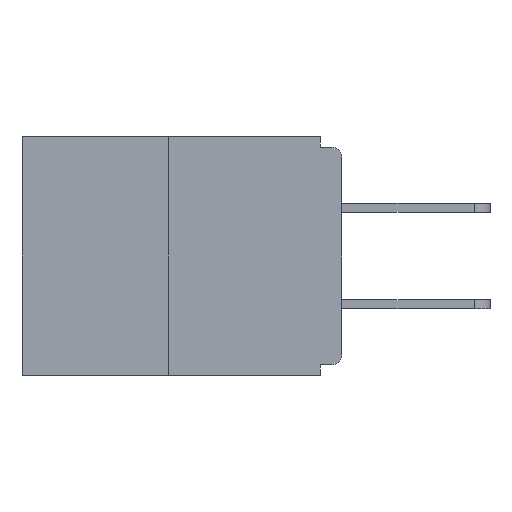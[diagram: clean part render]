
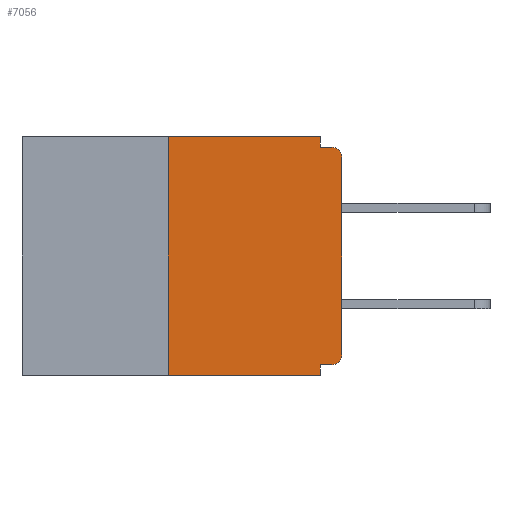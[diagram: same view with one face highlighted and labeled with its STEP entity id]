
A CAD part, left-side view. The second image highlights one B-rep face of the part: STEP entity #7056.
In plain terms, the highlighted planar face has unit normal (-1, 0, 0).
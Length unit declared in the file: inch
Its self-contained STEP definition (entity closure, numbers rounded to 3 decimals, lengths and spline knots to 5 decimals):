
#125 = VECTOR ( 'NONE', #9593, 39.37008 ) ;
#135 = CARTESIAN_POINT ( 'NONE',  ( 0., 0.25, 0. ) ) ;
#153 = ORIENTED_EDGE ( 'NONE', *, *, #1214, .F. ) ;
#228 = DIRECTION ( 'NONE',  ( 0., 0., -1. ) ) ;
#579 = VECTOR ( 'NONE', #12752, 39.37008 ) ;
#724 = VECTOR ( 'NONE', #10527, 39.37008 ) ;
#832 = VERTEX_POINT ( 'NONE', #11267 ) ;
#1214 = EDGE_CURVE ( 'NONE', #10467, #2780, #9408, .T. ) ;
#1393 = VECTOR ( 'NONE', #11596, 39.37008 ) ;
#1569 = LINE ( 'NONE', #135, #125 ) ;
#1639 = DIRECTION ( 'NONE',  ( 0., 0., 1. ) ) ;
#1794 = LINE ( 'NONE', #10461, #1393 ) ;
#1989 = DIRECTION ( 'NONE',  ( -1., 0., 0. ) ) ;
#2055 = CARTESIAN_POINT ( 'NONE',  ( 0., 0.015, -0.313 ) ) ;
#2281 = CIRCLE ( 'NONE', #5100, 0.015 ) ;
#2361 = DIRECTION ( 'NONE',  ( 0., -1., 0. ) ) ;
#2468 = AXIS2_PLACEMENT_3D ( 'NONE', #14831, #2995, #228 ) ;
#2730 = LINE ( 'NONE', #7684, #6453 ) ;
#2750 = LINE ( 'NONE', #16014, #3166 ) ;
#2780 = VERTEX_POINT ( 'NONE', #13529 ) ;
#2788 = EDGE_CURVE ( 'NONE', #3386, #13767, #2750, .T. ) ;
#2995 = DIRECTION ( 'NONE',  ( 1., 0., 0. ) ) ;
#3166 = VECTOR ( 'NONE', #12101, 39.37008 ) ;
#3386 = VERTEX_POINT ( 'NONE', #16720 ) ;
#3722 = ORIENTED_EDGE ( 'NONE', *, *, #16289, .T. ) ;
#4090 = LINE ( 'NONE', #14051, #579 ) ;
#4142 = VERTEX_POINT ( 'NONE', #4400 ) ;
#4199 = DIRECTION ( 'NONE',  ( 0., 0., -1. ) ) ;
#4240 = CARTESIAN_POINT ( 'NONE',  ( 0., 0., 0. ) ) ;
#4400 = CARTESIAN_POINT ( 'NONE',  ( 0., 0., -0.313 ) ) ;
#4488 = CARTESIAN_POINT ( 'NONE',  ( 0., 0.25, 0. ) ) ;
#4684 = EDGE_CURVE ( 'NONE', #14948, #16537, #7152, .T. ) ;
#4693 = CARTESIAN_POINT ( 'NONE',  ( 0., 0.031, 0. ) ) ;
#4766 = AXIS2_PLACEMENT_3D ( 'NONE', #6915, #13514, #4199 ) ;
#4981 = EDGE_CURVE ( 'NONE', #10146, #4142, #2281, .T. ) ;
#5100 = AXIS2_PLACEMENT_3D ( 'NONE', #2055, #1989, #10998 ) ;
#5228 = ORIENTED_EDGE ( 'NONE', *, *, #10253, .F. ) ;
#5931 = EDGE_CURVE ( 'NONE', #832, #13767, #4090, .T. ) ;
#6453 = VECTOR ( 'NONE', #2361, 39.37008 ) ;
#6619 = EDGE_CURVE ( 'NONE', #10146, #3386, #1794, .T. ) ;
#6891 = LINE ( 'NONE', #4240, #16654 ) ;
#6915 = CARTESIAN_POINT ( 'NONE',  ( 0., 0.015, -0.03 ) ) ;
#7056 = ADVANCED_FACE ( 'NONE', ( #9811 ), #8267, .F. ) ;
#7152 = CIRCLE ( 'NONE', #4766, 0.015 ) ;
#7530 = ORIENTED_EDGE ( 'NONE', *, *, #6619, .F. ) ;
#7584 = CARTESIAN_POINT ( 'NONE',  ( 0., 0.015, -0.015 ) ) ;
#7684 = CARTESIAN_POINT ( 'NONE',  ( 0., 0., -0.015 ) ) ;
#7883 = ORIENTED_EDGE ( 'NONE', *, *, #5931, .T. ) ;
#8267 = PLANE ( 'NONE',  #2468 ) ;
#8385 = CARTESIAN_POINT ( 'NONE',  ( 0., 0.015, -0.328 ) ) ;
#8609 = CARTESIAN_POINT ( 'NONE',  ( 0., 0.031, -0.343 ) ) ;
#8750 = VECTOR ( 'NONE', #12485, 39.37008 ) ;
#8785 = EDGE_CURVE ( 'NONE', #2780, #13128, #11383, .T. ) ;
#9408 = LINE ( 'NONE', #15729, #724 ) ;
#9593 = DIRECTION ( 'NONE',  ( 0., 0., 1. ) ) ;
#9705 = EDGE_LOOP ( 'NONE', ( #153, #10388, #7883, #16944, #7530, #16387, #3722, #10690, #5228, #16508 ) ) ;
#9811 = FACE_OUTER_BOUND ( 'NONE', #9705, .T. ) ;
#9878 = CARTESIAN_POINT ( 'NONE',  ( 0., 0.031, -0.015 ) ) ;
#10146 = VERTEX_POINT ( 'NONE', #8385 ) ;
#10253 = EDGE_CURVE ( 'NONE', #13128, #16537, #2730, .T. ) ;
#10388 = ORIENTED_EDGE ( 'NONE', *, *, #14535, .F. ) ;
#10461 = CARTESIAN_POINT ( 'NONE',  ( 0., 0., -0.328 ) ) ;
#10467 = VERTEX_POINT ( 'NONE', #4488 ) ;
#10527 = DIRECTION ( 'NONE',  ( 0., -1., 0. ) ) ;
#10690 = ORIENTED_EDGE ( 'NONE', *, *, #4684, .T. ) ;
#10998 = DIRECTION ( 'NONE',  ( 0., 0., -1. ) ) ;
#11267 = CARTESIAN_POINT ( 'NONE',  ( 0., 0.25, -0.343 ) ) ;
#11383 = LINE ( 'NONE', #4693, #8750 ) ;
#11596 = DIRECTION ( 'NONE',  ( 0., 1., 0. ) ) ;
#12101 = DIRECTION ( 'NONE',  ( 0., 0., -1. ) ) ;
#12485 = DIRECTION ( 'NONE',  ( 0., 0., -1. ) ) ;
#12628 = CARTESIAN_POINT ( 'NONE',  ( 0., 0., -0.03 ) ) ;
#12752 = DIRECTION ( 'NONE',  ( 0., -1., 0. ) ) ;
#13128 = VERTEX_POINT ( 'NONE', #9878 ) ;
#13514 = DIRECTION ( 'NONE',  ( -1., 0., 0. ) ) ;
#13529 = CARTESIAN_POINT ( 'NONE',  ( 0., 0.031, 0. ) ) ;
#13767 = VERTEX_POINT ( 'NONE', #8609 ) ;
#14051 = CARTESIAN_POINT ( 'NONE',  ( 0., 0.46, -0.343 ) ) ;
#14535 = EDGE_CURVE ( 'NONE', #832, #10467, #1569, .T. ) ;
#14831 = CARTESIAN_POINT ( 'NONE',  ( 0., 0.46, 0. ) ) ;
#14948 = VERTEX_POINT ( 'NONE', #12628 ) ;
#15729 = CARTESIAN_POINT ( 'NONE',  ( 0., 0.46, 0. ) ) ;
#16014 = CARTESIAN_POINT ( 'NONE',  ( 0., 0.031, -0.343 ) ) ;
#16289 = EDGE_CURVE ( 'NONE', #4142, #14948, #6891, .T. ) ;
#16387 = ORIENTED_EDGE ( 'NONE', *, *, #4981, .T. ) ;
#16508 = ORIENTED_EDGE ( 'NONE', *, *, #8785, .F. ) ;
#16537 = VERTEX_POINT ( 'NONE', #7584 ) ;
#16654 = VECTOR ( 'NONE', #1639, 39.37008 ) ;
#16720 = CARTESIAN_POINT ( 'NONE',  ( 0., 0.031, -0.328 ) ) ;
#16944 = ORIENTED_EDGE ( 'NONE', *, *, #2788, .F. ) ;
